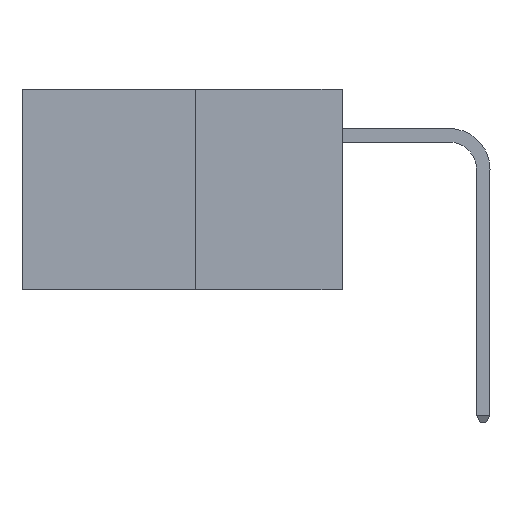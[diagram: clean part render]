
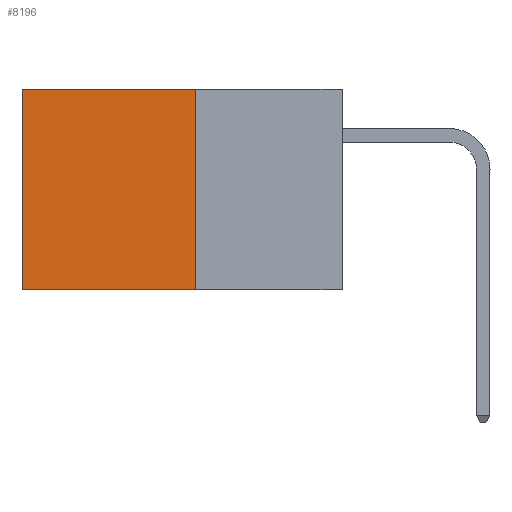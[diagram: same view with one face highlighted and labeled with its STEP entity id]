
A CAD part, left-side view. The second image highlights one B-rep face of the part: STEP entity #8196.
In plain terms, the highlighted planar face has unit normal (-1, 0, 0).
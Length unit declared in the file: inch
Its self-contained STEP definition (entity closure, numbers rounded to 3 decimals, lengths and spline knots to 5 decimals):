
#663 = DIRECTION ( 'NONE',  ( 0., 0., -1. ) ) ;
#2165 = CARTESIAN_POINT ( 'NONE',  ( 0.277, 0.59, -0.37 ) ) ;
#2660 = DIRECTION ( 'NONE',  ( 0., 1., 0. ) ) ;
#2707 = CARTESIAN_POINT ( 'NONE',  ( 0.277, 0.27, 0. ) ) ;
#2918 = EDGE_CURVE ( 'NONE', #8306, #4181, #15490, .T. ) ;
#3375 = VERTEX_POINT ( 'NONE', #10543 ) ;
#4181 = VERTEX_POINT ( 'NONE', #20046 ) ;
#6335 = VECTOR ( 'NONE', #663, 39.37008 ) ;
#6680 = FACE_OUTER_BOUND ( 'NONE', #8766, .T. ) ;
#7144 = CARTESIAN_POINT ( 'NONE',  ( 0.277, 0.27, -0.37 ) ) ;
#7287 = ORIENTED_EDGE ( 'NONE', *, *, #10886, .T. ) ;
#8196 = ADVANCED_FACE ( 'NONE', ( #6680 ), #15014, .F. ) ;
#8306 = VERTEX_POINT ( 'NONE', #15537 ) ;
#8353 = ORIENTED_EDGE ( 'NONE', *, *, #20527, .F. ) ;
#8577 = CARTESIAN_POINT ( 'NONE',  ( 0.277, 0.27, -0.37 ) ) ;
#8766 = EDGE_LOOP ( 'NONE', ( #16254, #8353, #10469, #7287 ) ) ;
#9466 = DIRECTION ( 'NONE',  ( 0., 0., -1. ) ) ;
#9904 = AXIS2_PLACEMENT_3D ( 'NONE', #7144, #15222, #15924 ) ;
#10469 = ORIENTED_EDGE ( 'NONE', *, *, #2918, .F. ) ;
#10543 = CARTESIAN_POINT ( 'NONE',  ( 0.277, 0.59, 0. ) ) ;
#10886 = EDGE_CURVE ( 'NONE', #8306, #3375, #11881, .T. ) ;
#10897 = LINE ( 'NONE', #17813, #6335 ) ;
#11366 = VECTOR ( 'NONE', #2660, 39.37008 ) ;
#11881 = LINE ( 'NONE', #2707, #11366 ) ;
#15014 = PLANE ( 'NONE',  #9904 ) ;
#15222 = DIRECTION ( 'NONE',  ( 1., 0., 0. ) ) ;
#15490 = LINE ( 'NONE', #8577, #19447 ) ;
#15537 = CARTESIAN_POINT ( 'NONE',  ( 0.277, 0.27, 0. ) ) ;
#15599 = VECTOR ( 'NONE', #19670, 39.37008 ) ;
#15924 = DIRECTION ( 'NONE',  ( 0., 0., -1. ) ) ;
#16136 = LINE ( 'NONE', #17957, #15599 ) ;
#16254 = ORIENTED_EDGE ( 'NONE', *, *, #19375, .T. ) ;
#17813 = CARTESIAN_POINT ( 'NONE',  ( 0.277, 0.59, -0.37 ) ) ;
#17928 = VERTEX_POINT ( 'NONE', #2165 ) ;
#17957 = CARTESIAN_POINT ( 'NONE',  ( 0.277, 0.27, -0.37 ) ) ;
#19375 = EDGE_CURVE ( 'NONE', #3375, #17928, #10897, .T. ) ;
#19447 = VECTOR ( 'NONE', #9466, 39.37008 ) ;
#19670 = DIRECTION ( 'NONE',  ( 0., 1., 0. ) ) ;
#20046 = CARTESIAN_POINT ( 'NONE',  ( 0.277, 0.27, -0.37 ) ) ;
#20527 = EDGE_CURVE ( 'NONE', #4181, #17928, #16136, .T. ) ;
